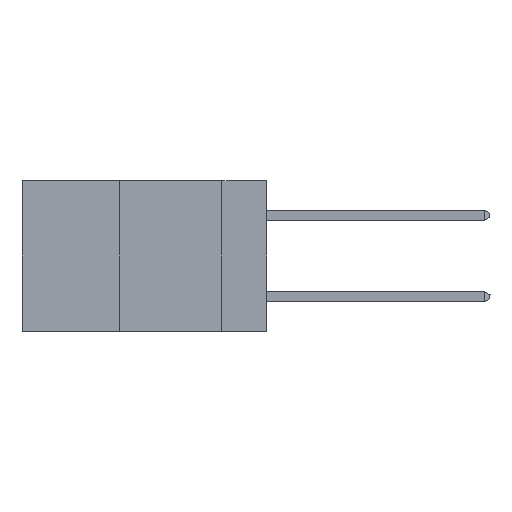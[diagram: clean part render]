
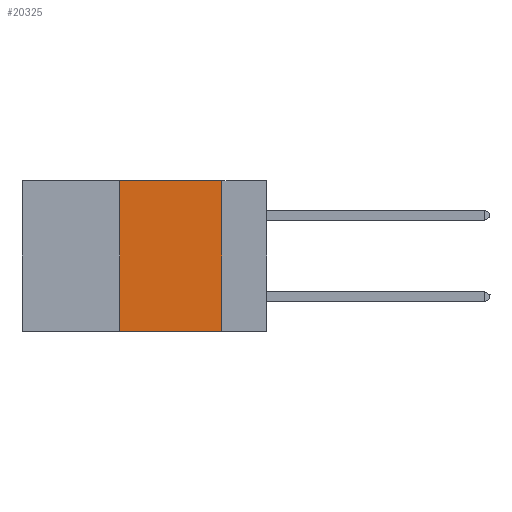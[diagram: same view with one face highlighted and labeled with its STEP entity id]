
A CAD part, left-side view. The second image highlights one B-rep face of the part: STEP entity #20325.
In plain terms, the highlighted planar face has unit normal (-1, 0, 0).
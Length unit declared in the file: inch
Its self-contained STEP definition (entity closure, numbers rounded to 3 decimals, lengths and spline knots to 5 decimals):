
#29 = VERTEX_POINT ( 'NONE', #24241 ) ;
#46 = LINE ( 'NONE', #8970, #31193 ) ;
#1705 = CARTESIAN_POINT ( 'NONE',  ( 0., 0.11, -0.37 ) ) ;
#3905 = EDGE_CURVE ( 'NONE', #41661, #29, #35951, .T. ) ;
#8196 = DIRECTION ( 'NONE',  ( 1., 0., 0. ) ) ;
#8970 = CARTESIAN_POINT ( 'NONE',  ( 0., 0.6, 0. ) ) ;
#9410 = CARTESIAN_POINT ( 'NONE',  ( 0., 0.36, -0.37 ) ) ;
#9914 = VECTOR ( 'NONE', #31300, 39.37008 ) ;
#10875 = EDGE_CURVE ( 'NONE', #41661, #23275, #39793, .T. ) ;
#12282 = DIRECTION ( 'NONE',  ( 0., -1., 0. ) ) ;
#13321 = ORIENTED_EDGE ( 'NONE', *, *, #3905, .F. ) ;
#13654 = FACE_OUTER_BOUND ( 'NONE', #30059, .T. ) ;
#16477 = DIRECTION ( 'NONE',  ( 0., 0., -1. ) ) ;
#16948 = EDGE_CURVE ( 'NONE', #18876, #23275, #29027, .T. ) ;
#17415 = ORIENTED_EDGE ( 'NONE', *, *, #16948, .F. ) ;
#18876 = VERTEX_POINT ( 'NONE', #41747 ) ;
#19303 = VECTOR ( 'NONE', #16477, 39.37008 ) ;
#20325 = ADVANCED_FACE ( 'NONE', ( #13654 ), #30898, .F. ) ;
#20423 = VECTOR ( 'NONE', #27984, 39.37008 ) ;
#23275 = VERTEX_POINT ( 'NONE', #1705 ) ;
#24241 = CARTESIAN_POINT ( 'NONE',  ( 0., 0.36, 0. ) ) ;
#25241 = ORIENTED_EDGE ( 'NONE', *, *, #10875, .T. ) ;
#27505 = CARTESIAN_POINT ( 'NONE',  ( 0., 0.6, 0. ) ) ;
#27761 = ORIENTED_EDGE ( 'NONE', *, *, #32450, .F. ) ;
#27984 = DIRECTION ( 'NONE',  ( 0., -1., 0. ) ) ;
#29027 = LINE ( 'NONE', #32467, #19303 ) ;
#30059 = EDGE_LOOP ( 'NONE', ( #17415, #27761, #13321, #25241 ) ) ;
#30628 = DIRECTION ( 'NONE',  ( 0., 0., -1. ) ) ;
#30660 = CARTESIAN_POINT ( 'NONE',  ( 0., 0.6, -0.37 ) ) ;
#30898 = PLANE ( 'NONE',  #35064 ) ;
#31193 = VECTOR ( 'NONE', #12282, 39.37008 ) ;
#31300 = DIRECTION ( 'NONE',  ( 0., 0., 1. ) ) ;
#32450 = EDGE_CURVE ( 'NONE', #29, #18876, #46, .T. ) ;
#32467 = CARTESIAN_POINT ( 'NONE',  ( 0., 0.11, 0. ) ) ;
#35064 = AXIS2_PLACEMENT_3D ( 'NONE', #27505, #8196, #30628 ) ;
#35951 = LINE ( 'NONE', #40967, #9914 ) ;
#39793 = LINE ( 'NONE', #30660, #20423 ) ;
#40967 = CARTESIAN_POINT ( 'NONE',  ( 0., 0.36, 0. ) ) ;
#41661 = VERTEX_POINT ( 'NONE', #9410 ) ;
#41747 = CARTESIAN_POINT ( 'NONE',  ( 0., 0.11, 0. ) ) ;
